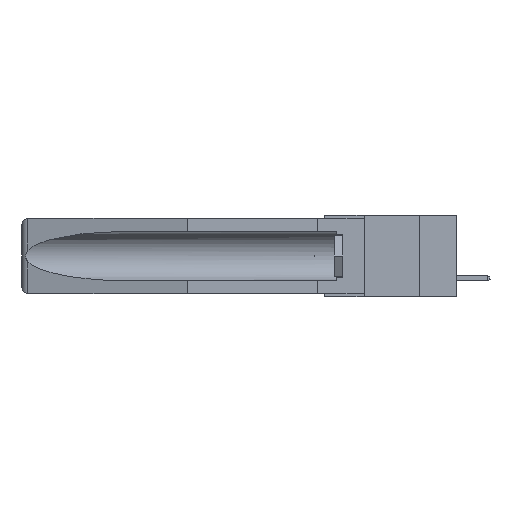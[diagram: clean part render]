
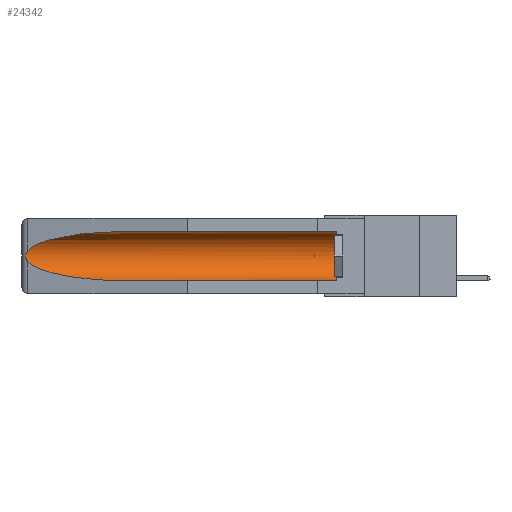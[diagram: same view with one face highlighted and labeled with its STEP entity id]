
A CAD part, left-side view. The second image highlights one B-rep face of the part: STEP entity #24342.
In plain terms, the highlighted cylindrical face has radius 2.857 mm (diameter 5.715 mm), a partial arc.
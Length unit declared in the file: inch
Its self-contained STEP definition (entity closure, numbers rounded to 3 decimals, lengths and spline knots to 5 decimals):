
#293 = ORIENTED_EDGE ( 'NONE', *, *, #2082, .T. ) ;
#312 = CARTESIAN_POINT ( 'NONE',  ( 0.26537, 1.52718, -0.14972 ) ) ;
#325 = CIRCLE ( 'NONE', #12691, 0.1125 ) ;
#1173 = CARTESIAN_POINT ( 'NONE',  ( 0.155, 0.126, -0.1715 ) ) ;
#1452 = CARTESIAN_POINT ( 'NONE',  ( 0.21114, 1.30732, -0.059 ) ) ;
#2082 = EDGE_CURVE ( 'NONE', #31615, #20532, #33611, .T. ) ;
#2092 = CARTESIAN_POINT ( 'NONE',  ( 0.26537, 1.52718, -0.19328 ) ) ;
#2431 =( BOUNDED_CURVE ( )  B_SPLINE_CURVE ( 3, ( #2092, #6880, #25185, #4919 ),
 .UNSPECIFIED., .F., .F. ) 
 B_SPLINE_CURVE_WITH_KNOTS ( ( 4, 4 ),
 ( 0.1948, 1.5708 ),
 .UNSPECIFIED. ) 
 CURVE ( )  GEOMETRIC_REPRESENTATION_ITEM ( )  RATIONAL_B_SPLINE_CURVE ( ( 1., 0.848, 0.848, 1. ) ) 
 REPRESENTATION_ITEM ( '' )  );
#3347 = EDGE_CURVE ( 'NONE', #20532, #28212, #2431, .T. ) ;
#3688 = ORIENTED_EDGE ( 'NONE', *, *, #17358, .T. ) ;
#3778 = DIRECTION ( 'NONE',  ( 0., 0., 1. ) ) ;
#3791 = CARTESIAN_POINT ( 'NONE',  ( 0.155, 1.07973, -0.284 ) ) ;
#4919 = CARTESIAN_POINT ( 'NONE',  ( 0.155, 1.07973, -0.284 ) ) ;
#5928 = LINE ( 'NONE', #21891, #30470 ) ;
#5958 = ORIENTED_EDGE ( 'NONE', *, *, #19130, .T. ) ;
#6880 = CARTESIAN_POINT ( 'NONE',  ( 0.25451, 1.48313, -0.24835 ) ) ;
#7834 = CARTESIAN_POINT ( 'NONE',  ( 0.155, 0.126, -0.059 ) ) ;
#8453 = VERTEX_POINT ( 'NONE', #7834 ) ;
#8818 = DIRECTION ( 'NONE',  ( 0., -1., 0. ) ) ;
#9319 = CARTESIAN_POINT ( 'NONE',  ( 0.26537, 1.52718, -0.14972 ) ) ;
#9405 = AXIS2_PLACEMENT_3D ( 'NONE', #9784, #12399, #30708 ) ;
#9654 = CARTESIAN_POINT ( 'NONE',  ( 0.26597, 1.5296, -0.19026 ) ) ;
#9784 = CARTESIAN_POINT ( 'NONE',  ( 0.155, -0.30754, -0.1715 ) ) ;
#10966 = ORIENTED_EDGE ( 'NONE', *, *, #3347, .T. ) ;
#12399 = DIRECTION ( 'NONE',  ( 0., 1., 0. ) ) ;
#12414 = VERTEX_POINT ( 'NONE', #21210 ) ;
#12691 = AXIS2_PLACEMENT_3D ( 'NONE', #1173, #8818, #3778 ) ;
#14560 = CARTESIAN_POINT ( 'NONE',  ( 0.155, 0.126, -0.284 ) ) ;
#14746 = CARTESIAN_POINT ( 'NONE',  ( 0.2673, 1.53269, -0.17917 ) ) ;
#15025 = VERTEX_POINT ( 'NONE', #14560 ) ;
#17015 = CARTESIAN_POINT ( 'NONE',  ( 0.26537, 1.52718, -0.14972 ) ) ;
#17358 = EDGE_CURVE ( 'NONE', #12414, #31615, #20616, .T. ) ;
#17826 = ORIENTED_EDGE ( 'NONE', *, *, #24881, .T. ) ;
#17888 = CYLINDRICAL_SURFACE ( 'NONE', #9405, 0.1125 ) ;
#19130 = EDGE_CURVE ( 'NONE', #8453, #12414, #24922, .T. ) ;
#20532 = VERTEX_POINT ( 'NONE', #30167 ) ;
#20616 =( BOUNDED_CURVE ( )  B_SPLINE_CURVE ( 3, ( #22227, #1452, #24984, #9319 ),
 .UNSPECIFIED., .F., .F. ) 
 B_SPLINE_CURVE_WITH_KNOTS ( ( 4, 4 ),
 ( 4.71239, 6.08839 ),
 .UNSPECIFIED. ) 
 CURVE ( )  GEOMETRIC_REPRESENTATION_ITEM ( )  RATIONAL_B_SPLINE_CURVE ( ( 1., 0.848, 0.848, 1. ) ) 
 REPRESENTATION_ITEM ( '' )  );
#21210 = CARTESIAN_POINT ( 'NONE',  ( 0.155, 1.07973, -0.059 ) ) ;
#21891 = CARTESIAN_POINT ( 'NONE',  ( 0.155, -0.30754, -0.284 ) ) ;
#22178 = EDGE_CURVE ( 'NONE', #15025, #28212, #5928, .T. ) ;
#22227 = CARTESIAN_POINT ( 'NONE',  ( 0.155, 1.07973, -0.059 ) ) ;
#22351 = CARTESIAN_POINT ( 'NONE',  ( 0.26537, 1.52718, -0.19328 ) ) ;
#23872 = CARTESIAN_POINT ( 'NONE',  ( 0.155, -0.30754, -0.059 ) ) ;
#24342 = ADVANCED_FACE ( 'NONE', ( #25308 ), #17888, .F. ) ;
#24881 = EDGE_CURVE ( 'NONE', #15025, #8453, #325, .T. ) ;
#24922 = LINE ( 'NONE', #23872, #31059 ) ;
#24984 = CARTESIAN_POINT ( 'NONE',  ( 0.25451, 1.48313, -0.09465 ) ) ;
#25185 = CARTESIAN_POINT ( 'NONE',  ( 0.21114, 1.30732, -0.284 ) ) ;
#25308 = FACE_OUTER_BOUND ( 'NONE', #33768, .T. ) ;
#25328 = CARTESIAN_POINT ( 'NONE',  ( 0.26654, 1.53092, -0.15636 ) ) ;
#27502 = ORIENTED_EDGE ( 'NONE', *, *, #22178, .F. ) ;
#27505 = DIRECTION ( 'NONE',  ( 0., 1., 0. ) ) ;
#27622 = CARTESIAN_POINT ( 'NONE',  ( 0.2675, 1.53308, -0.17534 ) ) ;
#28212 = VERTEX_POINT ( 'NONE', #3791 ) ;
#30167 = CARTESIAN_POINT ( 'NONE',  ( 0.26537, 1.52718, -0.19328 ) ) ;
#30229 = CARTESIAN_POINT ( 'NONE',  ( 0.26655, 1.53094, -0.18657 ) ) ;
#30457 = CARTESIAN_POINT ( 'NONE',  ( 0.2675, 1.53308, -0.16763 ) ) ;
#30470 = VECTOR ( 'NONE', #27505, 39.37008 ) ;
#30708 = DIRECTION ( 'NONE',  ( 0., 0., 1. ) ) ;
#31059 = VECTOR ( 'NONE', #31842, 39.37008 ) ;
#31615 = VERTEX_POINT ( 'NONE', #312 ) ;
#31842 = DIRECTION ( 'NONE',  ( 0., 1., 0. ) ) ;
#32707 = CARTESIAN_POINT ( 'NONE',  ( 0.26597, 1.52961, -0.15275 ) ) ;
#33052 = CARTESIAN_POINT ( 'NONE',  ( 0.2673, 1.5327, -0.16383 ) ) ;
#33611 = B_SPLINE_CURVE_WITH_KNOTS ( 'NONE', 3,
 ( #17015, #32707, #25328, #33052, #30457, #27622, #14746, #30229, #9654, #22351 ),
 .UNSPECIFIED., .F., .F.,
 ( 4, 2, 2, 2, 4 ),
 ( 0., 0.00029, 0.00058, 0.00087, 0.00117 ),
 .UNSPECIFIED. ) ;
#33768 = EDGE_LOOP ( 'NONE', ( #3688, #293, #10966, #27502, #17826, #5958 ) ) ;
